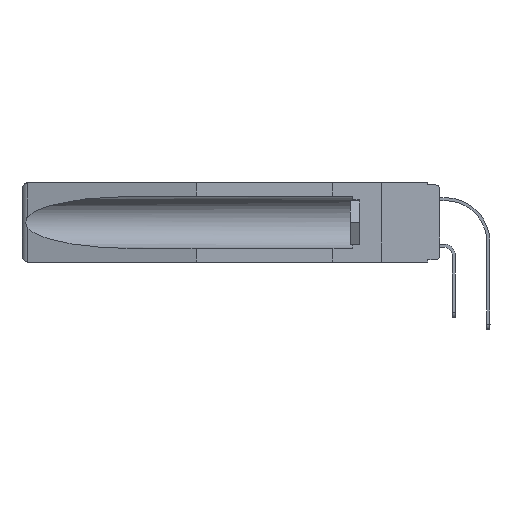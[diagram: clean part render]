
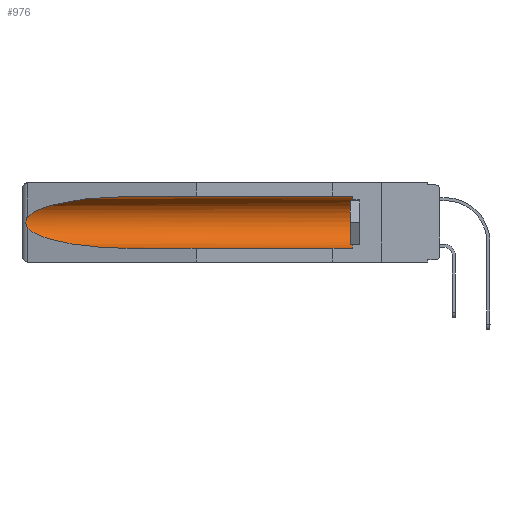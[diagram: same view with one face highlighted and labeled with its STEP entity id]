
A CAD part, left-side view. The second image highlights one B-rep face of the part: STEP entity #976.
In plain terms, the highlighted cylindrical face has radius 2.857 mm (diameter 5.715 mm), a partial arc.
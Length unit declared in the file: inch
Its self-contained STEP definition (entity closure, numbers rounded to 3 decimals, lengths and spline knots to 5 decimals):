
#203 = CARTESIAN_POINT ( 'NONE',  ( 0.26654, 1.53092, -0.15636 ) ) ;
#639 = ORIENTED_EDGE ( 'NONE', *, *, #10507, .T. ) ;
#897 = CARTESIAN_POINT ( 'NONE',  ( 0.155, 0.126, -0.059 ) ) ;
#976 = ADVANCED_FACE ( 'NONE', ( #14180 ), #4513, .F. ) ;
#1050 = DIRECTION ( 'NONE',  ( 0., -1., 0. ) ) ;
#1644 = ORIENTED_EDGE ( 'NONE', *, *, #12237, .T. ) ;
#2431 = DIRECTION ( 'NONE',  ( 0., 1., 0. ) ) ;
#2793 = CARTESIAN_POINT ( 'NONE',  ( 0.155, 0.126, -0.1715 ) ) ;
#4513 = CYLINDRICAL_SURFACE ( 'NONE', #6864, 0.1125 ) ;
#4960 = CARTESIAN_POINT ( 'NONE',  ( 0.155, -0.30754, -0.059 ) ) ;
#4975 = CARTESIAN_POINT ( 'NONE',  ( 0.155, 1.07973, -0.059 ) ) ;
#5059 = CARTESIAN_POINT ( 'NONE',  ( 0.21114, 1.30732, -0.284 ) ) ;
#5161 =( BOUNDED_CURVE ( )  B_SPLINE_CURVE ( 3, ( #4975, #16353, #10422, #6467 ),
 .UNSPECIFIED., .F., .F. ) 
 B_SPLINE_CURVE_WITH_KNOTS ( ( 4, 4 ),
 ( 4.71239, 6.08839 ),
 .UNSPECIFIED. ) 
 CURVE ( )  GEOMETRIC_REPRESENTATION_ITEM ( )  RATIONAL_B_SPLINE_CURVE ( ( 1., 0.848, 0.848, 1. ) ) 
 REPRESENTATION_ITEM ( '' )  );
#5437 = CIRCLE ( 'NONE', #14516, 0.1125 ) ;
#5767 = VECTOR ( 'NONE', #7255, 39.37008 ) ;
#5886 = CARTESIAN_POINT ( 'NONE',  ( 0.26597, 1.5296, -0.19026 ) ) ;
#6143 = CARTESIAN_POINT ( 'NONE',  ( 0.26537, 1.52718, -0.19328 ) ) ;
#6467 = CARTESIAN_POINT ( 'NONE',  ( 0.26537, 1.52718, -0.14972 ) ) ;
#6555 = CARTESIAN_POINT ( 'NONE',  ( 0.155, 1.07973, -0.284 ) ) ;
#6742 = CARTESIAN_POINT ( 'NONE',  ( 0.155, -0.30754, -0.1715 ) ) ;
#6864 = AXIS2_PLACEMENT_3D ( 'NONE', #6742, #2431, #8599 ) ;
#7255 = DIRECTION ( 'NONE',  ( 0., 1., 0. ) ) ;
#7749 = CARTESIAN_POINT ( 'NONE',  ( 0.2675, 1.53308, -0.17534 ) ) ;
#8343 = EDGE_CURVE ( 'NONE', #23957, #18178, #16336, .T. ) ;
#8599 = DIRECTION ( 'NONE',  ( 0., 0., 1. ) ) ;
#9078 = ORIENTED_EDGE ( 'NONE', *, *, #21257, .T. ) ;
#9474 =( BOUNDED_CURVE ( )  B_SPLINE_CURVE ( 3, ( #23466, #16075, #5059, #6555 ),
 .UNSPECIFIED., .F., .F. ) 
 B_SPLINE_CURVE_WITH_KNOTS ( ( 4, 4 ),
 ( 0.1948, 1.5708 ),
 .UNSPECIFIED. ) 
 CURVE ( )  GEOMETRIC_REPRESENTATION_ITEM ( )  RATIONAL_B_SPLINE_CURVE ( ( 1., 0.848, 0.848, 1. ) ) 
 REPRESENTATION_ITEM ( '' )  );
#9482 = CARTESIAN_POINT ( 'NONE',  ( 0.155, 1.07973, -0.284 ) ) ;
#10334 = EDGE_CURVE ( 'NONE', #10569, #16216, #18964, .T. ) ;
#10422 = CARTESIAN_POINT ( 'NONE',  ( 0.25451, 1.48313, -0.09465 ) ) ;
#10507 = EDGE_CURVE ( 'NONE', #12771, #23957, #5437, .T. ) ;
#10569 = VERTEX_POINT ( 'NONE', #18853 ) ;
#10699 = DIRECTION ( 'NONE',  ( 0., 0., 1. ) ) ;
#11020 = EDGE_LOOP ( 'NONE', ( #1644, #19867, #9078, #23049, #639, #21019 ) ) ;
#11185 = CARTESIAN_POINT ( 'NONE',  ( 0.155, 0.126, -0.284 ) ) ;
#12237 = EDGE_CURVE ( 'NONE', #18178, #10569, #5161, .T. ) ;
#12524 = DIRECTION ( 'NONE',  ( 0., 1., 0. ) ) ;
#12771 = VERTEX_POINT ( 'NONE', #11185 ) ;
#13751 = CARTESIAN_POINT ( 'NONE',  ( 0.155, 1.07973, -0.059 ) ) ;
#13784 = CARTESIAN_POINT ( 'NONE',  ( 0.26537, 1.52718, -0.19328 ) ) ;
#13810 = CARTESIAN_POINT ( 'NONE',  ( 0.26597, 1.52961, -0.15275 ) ) ;
#14180 = FACE_OUTER_BOUND ( 'NONE', #11020, .T. ) ;
#14516 = AXIS2_PLACEMENT_3D ( 'NONE', #2793, #1050, #10699 ) ;
#14930 = VECTOR ( 'NONE', #12524, 39.37008 ) ;
#15054 = CARTESIAN_POINT ( 'NONE',  ( 0.155, -0.30754, -0.284 ) ) ;
#15285 = CARTESIAN_POINT ( 'NONE',  ( 0.2673, 1.53269, -0.17917 ) ) ;
#15530 = CARTESIAN_POINT ( 'NONE',  ( 0.2673, 1.5327, -0.16383 ) ) ;
#15662 = CARTESIAN_POINT ( 'NONE',  ( 0.26537, 1.52718, -0.14972 ) ) ;
#16075 = CARTESIAN_POINT ( 'NONE',  ( 0.25451, 1.48313, -0.24835 ) ) ;
#16216 = VERTEX_POINT ( 'NONE', #13784 ) ;
#16336 = LINE ( 'NONE', #4960, #14930 ) ;
#16353 = CARTESIAN_POINT ( 'NONE',  ( 0.21114, 1.30732, -0.059 ) ) ;
#16913 = LINE ( 'NONE', #15054, #5767 ) ;
#17402 = CARTESIAN_POINT ( 'NONE',  ( 0.26655, 1.53094, -0.18657 ) ) ;
#18178 = VERTEX_POINT ( 'NONE', #13751 ) ;
#18853 = CARTESIAN_POINT ( 'NONE',  ( 0.26537, 1.52718, -0.14972 ) ) ;
#18964 = B_SPLINE_CURVE_WITH_KNOTS ( 'NONE', 3,
 ( #15662, #13810, #203, #15530, #22814, #7749, #15285, #17402, #5886, #6143 ),
 .UNSPECIFIED., .F., .F.,
 ( 4, 2, 2, 2, 4 ),
 ( 0., 0.00029, 0.00058, 0.00087, 0.00117 ),
 .UNSPECIFIED. ) ;
#19867 = ORIENTED_EDGE ( 'NONE', *, *, #10334, .T. ) ;
#21019 = ORIENTED_EDGE ( 'NONE', *, *, #8343, .T. ) ;
#21257 = EDGE_CURVE ( 'NONE', #16216, #23071, #9474, .T. ) ;
#22814 = CARTESIAN_POINT ( 'NONE',  ( 0.2675, 1.53308, -0.16763 ) ) ;
#23049 = ORIENTED_EDGE ( 'NONE', *, *, #23100, .F. ) ;
#23071 = VERTEX_POINT ( 'NONE', #9482 ) ;
#23100 = EDGE_CURVE ( 'NONE', #12771, #23071, #16913, .T. ) ;
#23466 = CARTESIAN_POINT ( 'NONE',  ( 0.26537, 1.52718, -0.19328 ) ) ;
#23957 = VERTEX_POINT ( 'NONE', #897 ) ;
